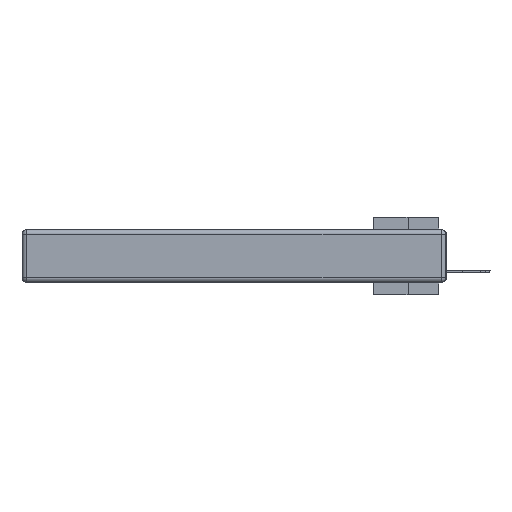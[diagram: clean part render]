
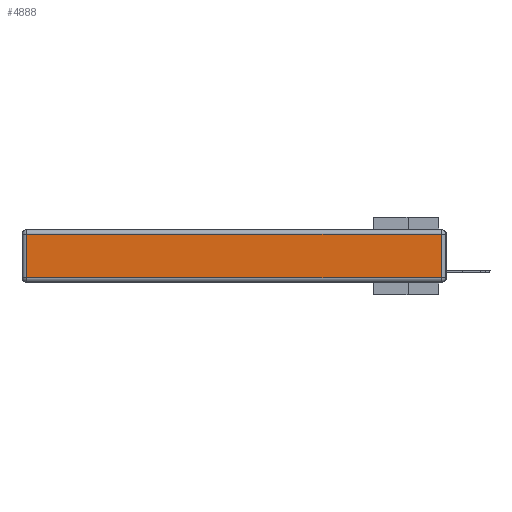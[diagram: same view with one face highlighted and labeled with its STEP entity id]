
A CAD part, left-side view. The second image highlights one B-rep face of the part: STEP entity #4888.
In plain terms, the highlighted planar face has unit normal (-1, 0, 0).
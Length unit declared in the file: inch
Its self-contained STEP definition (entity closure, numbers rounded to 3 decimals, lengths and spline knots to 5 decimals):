
#1009 = EDGE_CURVE ( 'NONE', #31735, #30717, #7427, .T. ) ;
#3997 = CARTESIAN_POINT ( 'NONE',  ( 0., 0.03, -0.03 ) ) ;
#4470 = DIRECTION ( 'NONE',  ( 0., 0., 1. ) ) ;
#4694 = DIRECTION ( 'NONE',  ( 0., 1., 0. ) ) ;
#4888 = ADVANCED_FACE ( 'NONE', ( #14055 ), #10839, .T. ) ;
#6499 = CARTESIAN_POINT ( 'NONE',  ( 0., 2.72, -0.03 ) ) ;
#7427 = LINE ( 'NONE', #34581, #32436 ) ;
#7674 = LINE ( 'NONE', #32041, #17404 ) ;
#10030 = CARTESIAN_POINT ( 'NONE',  ( 0., 2.72, -0.343 ) ) ;
#10635 = VECTOR ( 'NONE', #16371, 39.37008 ) ;
#10736 = EDGE_CURVE ( 'NONE', #20617, #23329, #38181, .T. ) ;
#10839 = PLANE ( 'NONE',  #29690 ) ;
#10968 = LINE ( 'NONE', #32545, #10635 ) ;
#14055 = FACE_OUTER_BOUND ( 'NONE', #18549, .T. ) ;
#16371 = DIRECTION ( 'NONE',  ( 0., -1., 0. ) ) ;
#16772 = ORIENTED_EDGE ( 'NONE', *, *, #39491, .T. ) ;
#16842 = CARTESIAN_POINT ( 'NONE',  ( 0., 0., -0.343 ) ) ;
#17404 = VECTOR ( 'NONE', #4694, 39.37008 ) ;
#18549 = EDGE_LOOP ( 'NONE', ( #16772, #25975, #20654, #22831 ) ) ;
#18825 = CARTESIAN_POINT ( 'NONE',  ( 0., 2.72, -0.313 ) ) ;
#19537 = EDGE_CURVE ( 'NONE', #30717, #20617, #7674, .T. ) ;
#20617 = VERTEX_POINT ( 'NONE', #6499 ) ;
#20654 = ORIENTED_EDGE ( 'NONE', *, *, #19537, .T. ) ;
#22831 = ORIENTED_EDGE ( 'NONE', *, *, #10736, .T. ) ;
#23329 = VERTEX_POINT ( 'NONE', #18825 ) ;
#25975 = ORIENTED_EDGE ( 'NONE', *, *, #1009, .T. ) ;
#28793 = DIRECTION ( 'NONE',  ( 0., 0., -1. ) ) ;
#29026 = DIRECTION ( 'NONE',  ( -1., 0., 0. ) ) ;
#29462 = CARTESIAN_POINT ( 'NONE',  ( 0., 0.03, -0.313 ) ) ;
#29690 = AXIS2_PLACEMENT_3D ( 'NONE', #16842, #29026, #4470 ) ;
#30717 = VERTEX_POINT ( 'NONE', #3997 ) ;
#31735 = VERTEX_POINT ( 'NONE', #29462 ) ;
#32041 = CARTESIAN_POINT ( 'NONE',  ( 0., 2.75, -0.03 ) ) ;
#32436 = VECTOR ( 'NONE', #35172, 39.37008 ) ;
#32545 = CARTESIAN_POINT ( 'NONE',  ( 0., 0., -0.313 ) ) ;
#34581 = CARTESIAN_POINT ( 'NONE',  ( 0., 0.03, -0.343 ) ) ;
#35172 = DIRECTION ( 'NONE',  ( 0., 0., 1. ) ) ;
#35390 = VECTOR ( 'NONE', #28793, 39.37008 ) ;
#38181 = LINE ( 'NONE', #10030, #35390 ) ;
#39491 = EDGE_CURVE ( 'NONE', #23329, #31735, #10968, .T. ) ;
